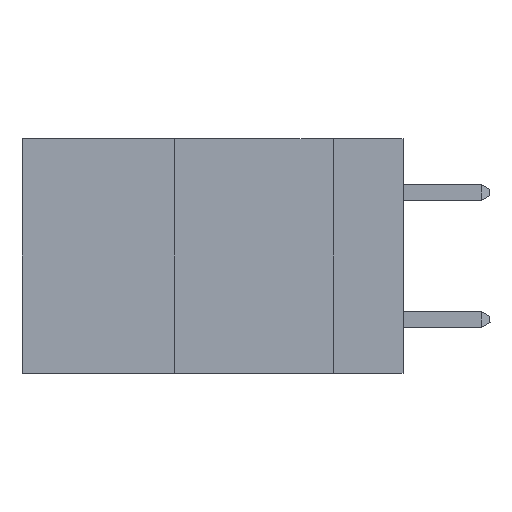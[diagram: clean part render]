
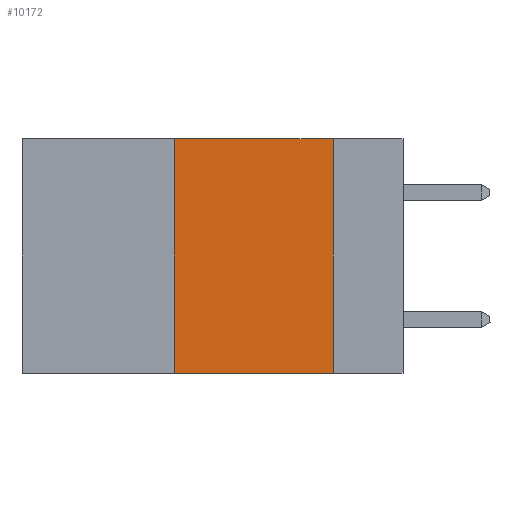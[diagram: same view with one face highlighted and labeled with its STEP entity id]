
A CAD part, left-side view. The second image highlights one B-rep face of the part: STEP entity #10172.
In plain terms, the highlighted planar face has unit normal (-1, 0, 0).
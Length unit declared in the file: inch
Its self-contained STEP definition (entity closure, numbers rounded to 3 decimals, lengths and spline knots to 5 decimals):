
#1334 = DIRECTION ( 'NONE',  ( 0., 0., 1. ) ) ;
#1471 = VERTEX_POINT ( 'NONE', #10012 ) ;
#1504 = VECTOR ( 'NONE', #16754, 39.37008 ) ;
#2553 = ORIENTED_EDGE ( 'NONE', *, *, #10886, .F. ) ;
#2600 = DIRECTION ( 'NONE',  ( 1., 0., 0. ) ) ;
#2801 = DIRECTION ( 'NONE',  ( 0., 0., -1. ) ) ;
#3864 = VECTOR ( 'NONE', #1334, 39.37008 ) ;
#5165 = VECTOR ( 'NONE', #2801, 39.37008 ) ;
#5289 = EDGE_CURVE ( 'NONE', #8409, #1471, #12705, .T. ) ;
#5381 = ORIENTED_EDGE ( 'NONE', *, *, #5410, .T. ) ;
#5410 = EDGE_CURVE ( 'NONE', #8409, #15949, #19949, .T. ) ;
#5463 = CARTESIAN_POINT ( 'NONE',  ( 0., 0.11, -0.37 ) ) ;
#5465 = DIRECTION ( 'NONE',  ( 0., -1., 0. ) ) ;
#7225 = EDGE_CURVE ( 'NONE', #1471, #18050, #13153, .T. ) ;
#7685 = CARTESIAN_POINT ( 'NONE',  ( 0., 0.36, 0. ) ) ;
#8358 = AXIS2_PLACEMENT_3D ( 'NONE', #19002, #2600, #10697 ) ;
#8409 = VERTEX_POINT ( 'NONE', #20664 ) ;
#8787 = CARTESIAN_POINT ( 'NONE',  ( 0., 0.11, 0. ) ) ;
#10012 = CARTESIAN_POINT ( 'NONE',  ( 0., 0.36, 0. ) ) ;
#10172 = ADVANCED_FACE ( 'NONE', ( #15080 ), #15650, .F. ) ;
#10697 = DIRECTION ( 'NONE',  ( 0., 0., -1. ) ) ;
#10886 = EDGE_CURVE ( 'NONE', #18050, #15949, #19507, .T. ) ;
#12705 = LINE ( 'NONE', #7685, #3864 ) ;
#13153 = LINE ( 'NONE', #20107, #1504 ) ;
#15080 = FACE_OUTER_BOUND ( 'NONE', #19271, .T. ) ;
#15650 = PLANE ( 'NONE',  #8358 ) ;
#15672 = ORIENTED_EDGE ( 'NONE', *, *, #5289, .F. ) ;
#15949 = VERTEX_POINT ( 'NONE', #5463 ) ;
#16754 = DIRECTION ( 'NONE',  ( 0., -1., 0. ) ) ;
#18050 = VERTEX_POINT ( 'NONE', #8787 ) ;
#18913 = CARTESIAN_POINT ( 'NONE',  ( 0., 0.6, -0.37 ) ) ;
#19002 = CARTESIAN_POINT ( 'NONE',  ( 0., 0.6, 0. ) ) ;
#19271 = EDGE_LOOP ( 'NONE', ( #2553, #20313, #15672, #5381 ) ) ;
#19507 = LINE ( 'NONE', #20943, #5165 ) ;
#19949 = LINE ( 'NONE', #18913, #20999 ) ;
#20107 = CARTESIAN_POINT ( 'NONE',  ( 0., 0.6, 0. ) ) ;
#20313 = ORIENTED_EDGE ( 'NONE', *, *, #7225, .F. ) ;
#20664 = CARTESIAN_POINT ( 'NONE',  ( 0., 0.36, -0.37 ) ) ;
#20943 = CARTESIAN_POINT ( 'NONE',  ( 0., 0.11, 0. ) ) ;
#20999 = VECTOR ( 'NONE', #5465, 39.37008 ) ;
